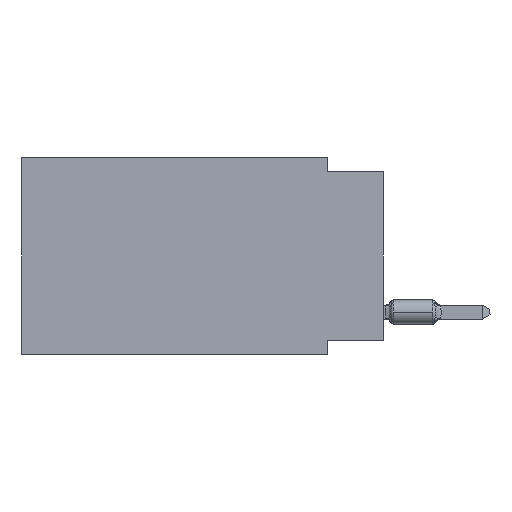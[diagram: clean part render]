
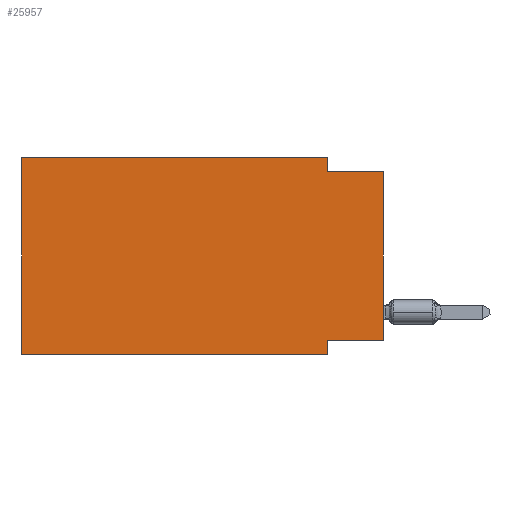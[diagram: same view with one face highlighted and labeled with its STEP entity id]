
A CAD part, left-side view. The second image highlights one B-rep face of the part: STEP entity #25957.
In plain terms, the highlighted planar face has unit normal (-1, 0, 0).
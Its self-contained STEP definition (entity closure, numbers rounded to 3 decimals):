
#257 = ORIENTED_EDGE ( 'NONE', *, *, #29934, .F. ) ;
#1406 = CARTESIAN_POINT ( 'NONE',  ( 0., 16.383, -8.89 ) ) ;
#1611 = ORIENTED_EDGE ( 'NONE', *, *, #24081, .F. ) ;
#2112 = DIRECTION ( 'NONE',  ( 0., 0., -1. ) ) ;
#2133 = EDGE_CURVE ( 'NONE', #18267, #15815, #21877, .T. ) ;
#2599 = VECTOR ( 'NONE', #6430, 1000. ) ;
#4213 = VERTEX_POINT ( 'NONE', #23445 ) ;
#4839 = LINE ( 'NONE', #14099, #5102 ) ;
#5102 = VECTOR ( 'NONE', #2112, 1000. ) ;
#5257 = PLANE ( 'NONE',  #16120 ) ;
#5596 = CARTESIAN_POINT ( 'NONE',  ( 0., 16.383, 0. ) ) ;
#6430 = DIRECTION ( 'NONE',  ( 0., 0., 1. ) ) ;
#7105 = CARTESIAN_POINT ( 'NONE',  ( 0., 0., -0.635 ) ) ;
#7397 = CARTESIAN_POINT ( 'NONE',  ( 0., 2.54, -8.89 ) ) ;
#7557 = FACE_OUTER_BOUND ( 'NONE', #8294, .T. ) ;
#7704 = DIRECTION ( 'NONE',  ( 0., 1., 0. ) ) ;
#7717 = LINE ( 'NONE', #5596, #28097 ) ;
#8294 = EDGE_LOOP ( 'NONE', ( #14815, #12707, #9499, #19333, #257, #20696, #1611, #21908 ) ) ;
#8931 = LINE ( 'NONE', #10623, #14014 ) ;
#9499 = ORIENTED_EDGE ( 'NONE', *, *, #24768, .F. ) ;
#10623 = CARTESIAN_POINT ( 'NONE',  ( 0., 16.383, 0. ) ) ;
#11197 = LINE ( 'NONE', #7105, #14142 ) ;
#11832 = CARTESIAN_POINT ( 'NONE',  ( 0., 2.54, -0.635 ) ) ;
#12408 = DIRECTION ( 'NONE',  ( 0., 0., -1. ) ) ;
#12707 = ORIENTED_EDGE ( 'NONE', *, *, #14962, .F. ) ;
#14014 = VECTOR ( 'NONE', #15905, 1000. ) ;
#14099 = CARTESIAN_POINT ( 'NONE',  ( 0., 2.54, -8.89 ) ) ;
#14142 = VECTOR ( 'NONE', #16354, 1000. ) ;
#14815 = ORIENTED_EDGE ( 'NONE', *, *, #18747, .T. ) ;
#14962 = EDGE_CURVE ( 'NONE', #16595, #15570, #11197, .T. ) ;
#15539 = VERTEX_POINT ( 'NONE', #21680 ) ;
#15570 = VERTEX_POINT ( 'NONE', #24255 ) ;
#15815 = VERTEX_POINT ( 'NONE', #7397 ) ;
#15838 = CARTESIAN_POINT ( 'NONE',  ( 0., 0., 0. ) ) ;
#15905 = DIRECTION ( 'NONE',  ( 0., -1., 0. ) ) ;
#16120 = AXIS2_PLACEMENT_3D ( 'NONE', #19523, #16942, #12408 ) ;
#16354 = DIRECTION ( 'NONE',  ( 0., -1., 0. ) ) ;
#16595 = VERTEX_POINT ( 'NONE', #11832 ) ;
#16827 = DIRECTION ( 'NONE',  ( 0., 0., 1. ) ) ;
#16942 = DIRECTION ( 'NONE',  ( 1., 0., 0. ) ) ;
#17403 = LINE ( 'NONE', #17549, #28320 ) ;
#17549 = CARTESIAN_POINT ( 'NONE',  ( 0., 0., -8.255 ) ) ;
#17817 = LINE ( 'NONE', #19663, #26463 ) ;
#18267 = VERTEX_POINT ( 'NONE', #1406 ) ;
#18747 = EDGE_CURVE ( 'NONE', #24836, #15570, #22817, .T. ) ;
#19133 = VERTEX_POINT ( 'NONE', #25536 ) ;
#19333 = ORIENTED_EDGE ( 'NONE', *, *, #29565, .F. ) ;
#19518 = CARTESIAN_POINT ( 'NONE',  ( 0., 0., -8.255 ) ) ;
#19523 = CARTESIAN_POINT ( 'NONE',  ( 0., 16.383, 0. ) ) ;
#19663 = CARTESIAN_POINT ( 'NONE',  ( 0., 2.54, 0. ) ) ;
#19734 = DIRECTION ( 'NONE',  ( 0., -1., 0. ) ) ;
#20098 = DIRECTION ( 'NONE',  ( 0., 0., -1. ) ) ;
#20696 = ORIENTED_EDGE ( 'NONE', *, *, #2133, .T. ) ;
#21202 = EDGE_CURVE ( 'NONE', #24836, #19133, #17403, .T. ) ;
#21680 = CARTESIAN_POINT ( 'NONE',  ( 0., 2.54, 0. ) ) ;
#21877 = LINE ( 'NONE', #22310, #25137 ) ;
#21908 = ORIENTED_EDGE ( 'NONE', *, *, #21202, .F. ) ;
#22310 = CARTESIAN_POINT ( 'NONE',  ( 0., 16.383, -8.89 ) ) ;
#22817 = LINE ( 'NONE', #15838, #2599 ) ;
#23445 = CARTESIAN_POINT ( 'NONE',  ( 0., 16.383, 0. ) ) ;
#24081 = EDGE_CURVE ( 'NONE', #19133, #15815, #4839, .T. ) ;
#24255 = CARTESIAN_POINT ( 'NONE',  ( 0., 0., -0.635 ) ) ;
#24768 = EDGE_CURVE ( 'NONE', #15539, #16595, #17817, .T. ) ;
#24836 = VERTEX_POINT ( 'NONE', #19518 ) ;
#25137 = VECTOR ( 'NONE', #19734, 1000. ) ;
#25536 = CARTESIAN_POINT ( 'NONE',  ( 0., 2.54, -8.255 ) ) ;
#25957 = ADVANCED_FACE ( 'NONE', ( #7557 ), #5257, .F. ) ;
#26463 = VECTOR ( 'NONE', #20098, 1000. ) ;
#28097 = VECTOR ( 'NONE', #16827, 1000. ) ;
#28320 = VECTOR ( 'NONE', #7704, 1000. ) ;
#29565 = EDGE_CURVE ( 'NONE', #4213, #15539, #8931, .T. ) ;
#29934 = EDGE_CURVE ( 'NONE', #18267, #4213, #7717, .T. ) ;
